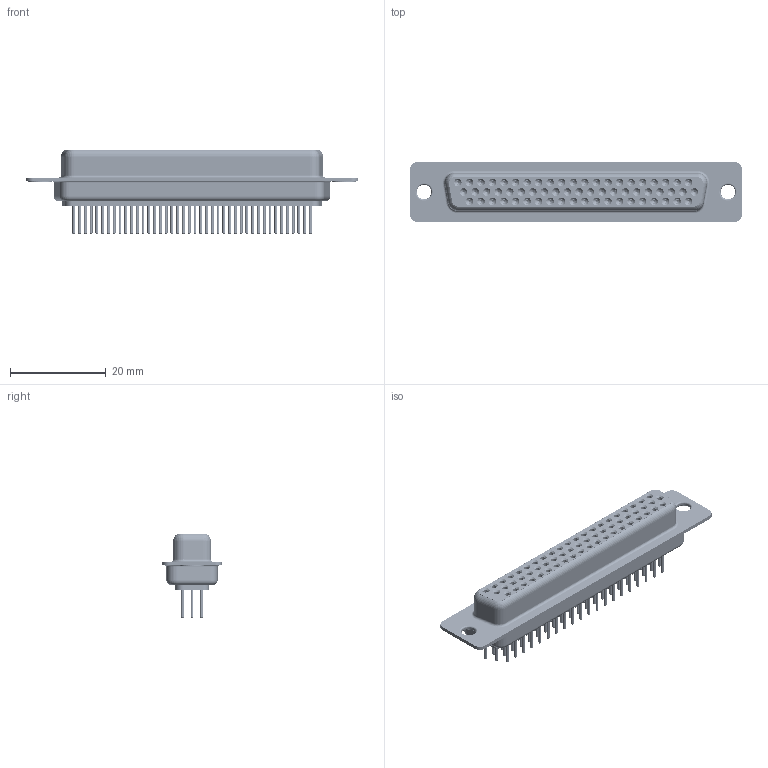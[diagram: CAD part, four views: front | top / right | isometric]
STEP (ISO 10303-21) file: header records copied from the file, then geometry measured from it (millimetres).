
FILE_DESCRIPTION (( 'STEP AP203' ), '1' );
FILE_NAME ('638-M62-230-BN1.STEP', '2022-07-05T21:04:28', ( '' ), ( '' ), 'SwSTEP 2.0', 'SolidWorks 2020', '' );
FILE_SCHEMA (( 'CONFIG_CONTROL_DESIGN' ));
Length unit declared in the file: millimetre
Products named in the file (8): 638M Contact Row 3_30; 638M Contact Row 2_30; 638M Shell Rear_62 Contacts; 638-M62-230-BN1; 638M Contact Row 1_30; 638M Thru Hole Rivet; 638M Housing_62 Contacts; 638M Shell Front_62 Contacts
Assembly tree (67 placements, depth 2):
  638-M62-230-BN1
    638M Housing_62 Contacts
    638M Shell Front_62 Contacts
    638M Shell Rear_62 Contacts
    638M Contact Row 1_30  x21
    638M Contact Row 2_30  x21
    638M Contact Row 3_30  x20
    638M Thru Hole Rivet  x2
Bounding box: 69.4 x 12.5 x 17.6 mm (x, y, z)
Volume: 4903.8 mm3; surface area: 16294.4 mm2
Topology: 67 solids, 67 shells, 3663 faces, 8415 edges, 5145 vertices
Faces by surface type: cylinder 1299, plane 997, torus 933, cone 434
Entity records: 35892 total; most frequent: DIRECTION 6567, CARTESIAN_POINT 5718, ORIENTED_EDGE 5174, AXIS2_PLACEMENT_3D 2814, EDGE_CURVE 2587, VERTEX_POINT 1640, CIRCLE 1579, EDGE_LOOP 1507
